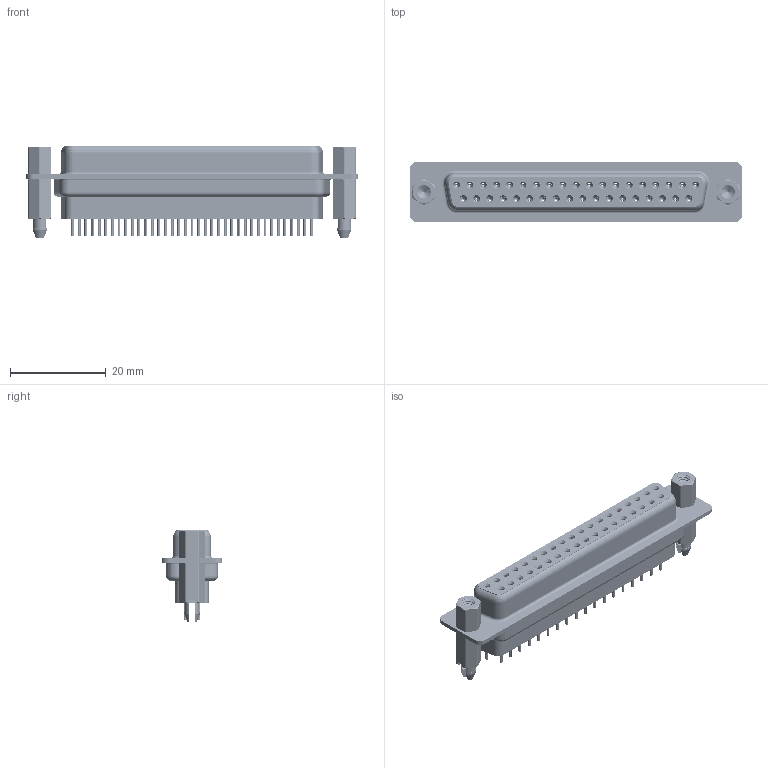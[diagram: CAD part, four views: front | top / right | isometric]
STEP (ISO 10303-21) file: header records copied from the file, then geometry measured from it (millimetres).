
FILE_DESCRIPTION (( 'STEP AP203' ), '1' );
FILE_NAME ('628-037-228-067.STEP', '2020-07-21T13:44:16', ( '' ), ( '' ), 'SwSTEP 2.0', 'SolidWorks 2020', '' );
FILE_SCHEMA (( 'CONFIG_CONTROL_DESIGN' ));
Length unit declared in the file: millimetre
Products named in the file (8): 628 Housing_37 FF; 628 4-40 Threaded Boardlock_FF; 628-037-228-067; 628 Contact Row 1_28L; 628 4-40 Hex Standoff; 628 Shell Front_37 Contacts; 628 Contact Row 2_28L; 628 Shell Rear_37 Contacts
Assembly tree (44 placements, depth 2):
  628-037-228-067
    628 Housing_37 FF
    628 Shell Front_37 Contacts
    628 Shell Rear_37 Contacts
    628 Contact Row 1_28L  x19
    628 Contact Row 2_28L  x18
    628 4-40 Hex Standoff  x2
    628 4-40 Threaded Boardlock_FF  x2
Bounding box: 69.3 x 12.6 x 19.4 mm (x, y, z)
Volume: 6613.6 mm3; surface area: 14924.4 mm2
Topology: 44 solids, 44 shells, 5260 faces, 13493 edges, 8404 vertices
Faces by surface type: cylinder 1496, plane 1268, torus 1025, bspline 806, cone 665
Entity records: 53759 total; most frequent: CARTESIAN_POINT 26428, DIRECTION 5475, ORIENTED_EDGE 5260, EDGE_CURVE 2630, AXIS2_PLACEMENT_3D 2276, VERTEX_POINT 1673, EDGE_LOOP 1301, CIRCLE 1210
